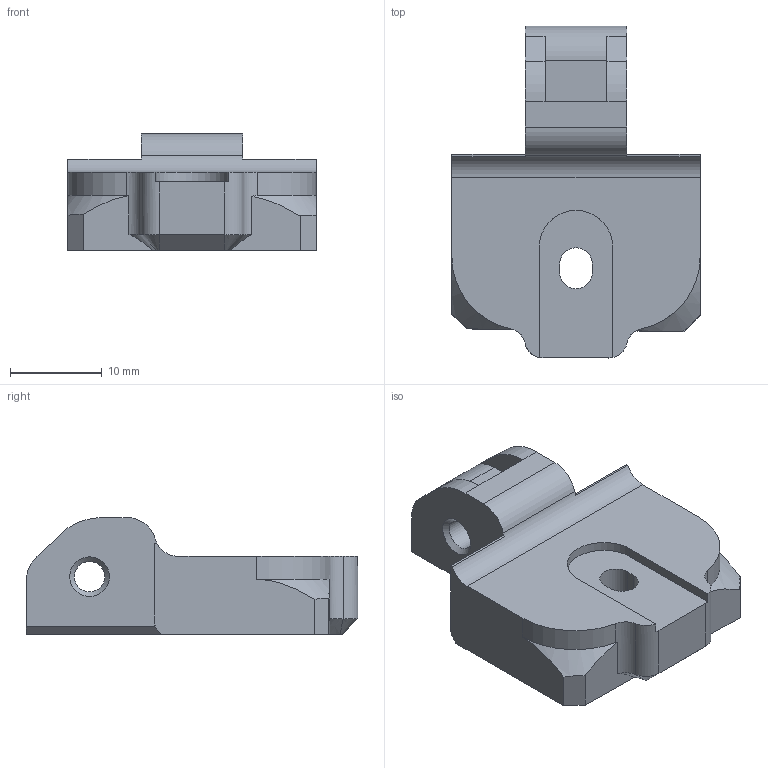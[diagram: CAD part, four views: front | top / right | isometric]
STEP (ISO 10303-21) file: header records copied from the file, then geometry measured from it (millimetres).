
FILE_DESCRIPTION(/* description */ ('STEP AP242','CAx-IF Rec.Pracs.---Representation and Presentation of Product Manufacturing Information (PMI)---4.0---2014-10-13','CAx-IF Rec.Pracs.---3D Tessellated Geometry---0.4---2014-09-14','2;1'),/* implementation_level */ '2;1');
FILE_NAME(/* name */ '62018eccb049f56281881075',/* time_stamp */ '2022-02-07T21:27:41+00:00',/* author */ (''),/* organization */ (''),/* preprocessor_version */ 'ST-DEVELOPER v18.101',/* originating_system */ ' ',/* authorisation */ ' ');
FILE_SCHEMA (('AP242_MANAGED_MODEL_BASED_3D_ENGINEERING_MIM_LF { 1 0 10303 442 1 1 4 }'));
Length unit declared in the file: metre
Products named in the file (1): Block (Print @ 99% Infill)
Bounding box: 27 x 36.09 x 12.7 mm (x, y, z)
Volume: 5876.6 mm3; surface area: 2728.5 mm2
Topology: 1 solids, 1 shells, 64 faces, 175 edges, 113 vertices
Faces by surface type: plane 35, cylinder 19, cone 8, torus 2
Full cylindrical faces by diameter (mm): 3.302 x1
Entity records: 2051 total; most frequent: CARTESIAN_POINT 394, ORIENTED_EDGE 342, DIRECTION 342, EDGE_CURVE 171, AXIS2_PLACEMENT_3D 119, VERTEX_POINT 112, LINE 104, VECTOR 104
